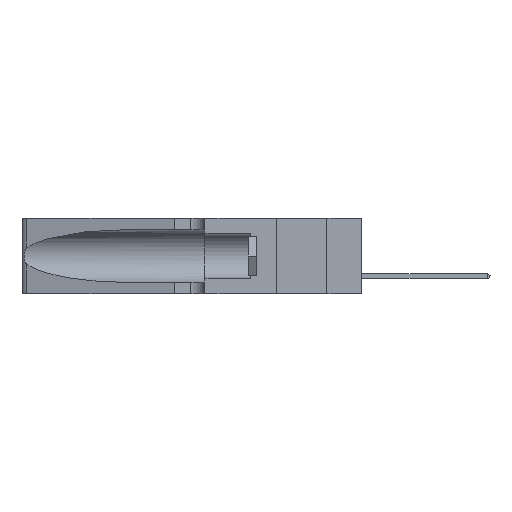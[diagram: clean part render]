
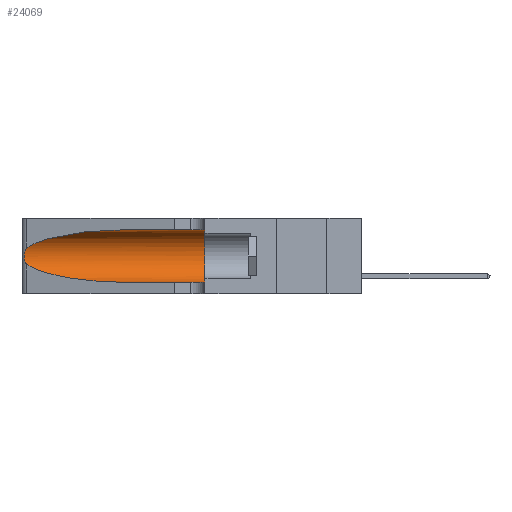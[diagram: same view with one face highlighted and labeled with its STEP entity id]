
A CAD part, left-side view. The second image highlights one B-rep face of the part: STEP entity #24069.
In plain terms, the highlighted cylindrical face has radius 3.308 mm (diameter 6.617 mm), a partial arc.
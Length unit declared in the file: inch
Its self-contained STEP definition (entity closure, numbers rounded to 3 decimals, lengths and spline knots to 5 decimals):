
#251 = CARTESIAN_POINT ( 'NONE',  ( 0.1305, 0.35, 0.05475 ) ) ;
#372 = LINE ( 'NONE', #10581, #31776 ) ;
#395 = VERTEX_POINT ( 'NONE', #18227 ) ;
#619 = CARTESIAN_POINT ( 'NONE',  ( 0.26017, 1.23833, 0.17102 ) ) ;
#1752 = VERTEX_POINT ( 'NONE', #15629 ) ;
#1945 = CARTESIAN_POINT ( 'NONE',  ( 0.25787, 1.23484, 0.2124 ) ) ;
#1964 =( BOUNDED_CURVE ( )  B_SPLINE_CURVE ( 3, ( #29571, #5136, #15035, #30301 ),
 .UNSPECIFIED., .F., .F. ) 
 B_SPLINE_CURVE_WITH_KNOTS ( ( 4, 4 ),
 ( 1.5708, 2.84003 ),
 .UNSPECIFIED. ) 
 CURVE ( )  GEOMETRIC_REPRESENTATION_ITEM ( )  RATIONAL_B_SPLINE_CURVE ( ( 1., 0.87, 0.87, 1. ) ) 
 REPRESENTATION_ITEM ( '' )  );
#4533 = ORIENTED_EDGE ( 'NONE', *, *, #20841, .F. ) ;
#4893 = VERTEX_POINT ( 'NONE', #251 ) ;
#5136 = CARTESIAN_POINT ( 'NONE',  ( 0.18966, 0.96281, 0.31525 ) ) ;
#5441 = AXIS2_PLACEMENT_3D ( 'NONE', #22650, #25826, #28469 ) ;
#7196 = CARTESIAN_POINT ( 'NONE',  ( 0.25555, 1.22994, 0.2215 ) ) ;
#7290 = DIRECTION ( 'NONE',  ( 0., -1., 0. ) ) ;
#7415 = VECTOR ( 'NONE', #7290, 39.37008 ) ;
#7799 = CARTESIAN_POINT ( 'NONE',  ( 0.25487, 1.22718, 0.14631 ) ) ;
#8104 = DIRECTION ( 'NONE',  ( 0., 1., 0. ) ) ;
#8957 = CARTESIAN_POINT ( 'NONE',  ( 0.1305, 0.72297, 0.05475 ) ) ;
#9062 = VERTEX_POINT ( 'NONE', #10924 ) ;
#9715 = VERTEX_POINT ( 'NONE', #16501 ) ;
#9868 = CYLINDRICAL_SURFACE ( 'NONE', #5441, 0.13025 ) ;
#10155 = CARTESIAN_POINT ( 'NONE',  ( 0.26018, 1.23835, 0.19895 ) ) ;
#10369 = CARTESIAN_POINT ( 'NONE',  ( 0.25639, 1.23186, 0.15144 ) ) ;
#10581 = CARTESIAN_POINT ( 'NONE',  ( 0.1305, 1.61858, 0.05475 ) ) ;
#10808 = ORIENTED_EDGE ( 'NONE', *, *, #13921, .T. ) ;
#10924 = CARTESIAN_POINT ( 'NONE',  ( 0.25487, 1.22718, 0.22369 ) ) ;
#11515 = CARTESIAN_POINT ( 'NONE',  ( 0.18966, 0.96281, 0.05475 ) ) ;
#12256 = B_SPLINE_CURVE_WITH_KNOTS ( 'NONE', 3,
 ( #16775, #7196, #29017, #1945, #22813, #10155, #22604, #27785, #619, #30407, #27897, #10369, #12957, #7799 ),
 .UNSPECIFIED., .F., .F.,
 ( 4, 2, 2, 2, 2, 2, 4 ),
 ( 0., 0.00027, 0.00053, 0.00107, 0.0016, 0.00187, 0.00214 ),
 .UNSPECIFIED. ) ;
#12534 = CARTESIAN_POINT ( 'NONE',  ( 0.1305, 1.61858, 0.31525 ) ) ;
#12957 = CARTESIAN_POINT ( 'NONE',  ( 0.25555, 1.22993, 0.14849 ) ) ;
#13382 = DIRECTION ( 'NONE',  ( 0., -1., 0. ) ) ;
#13627 = EDGE_CURVE ( 'NONE', #395, #9062, #1964, .T. ) ;
#13921 = EDGE_CURVE ( 'NONE', #1752, #9715, #23591, .T. ) ;
#14079 = CARTESIAN_POINT ( 'NONE',  ( 0.1305, 0.35, 0.31525 ) ) ;
#15035 = CARTESIAN_POINT ( 'NONE',  ( 0.2373, 1.15595, 0.28018 ) ) ;
#15629 = CARTESIAN_POINT ( 'NONE',  ( 0.25487, 1.22718, 0.14631 ) ) ;
#16501 = CARTESIAN_POINT ( 'NONE',  ( 0.1305, 0.72297, 0.05475 ) ) ;
#16662 = VERTEX_POINT ( 'NONE', #14079 ) ;
#16775 = CARTESIAN_POINT ( 'NONE',  ( 0.25487, 1.22718, 0.22369 ) ) ;
#17784 = ORIENTED_EDGE ( 'NONE', *, *, #29900, .T. ) ;
#18227 = CARTESIAN_POINT ( 'NONE',  ( 0.1305, 0.72297, 0.31525 ) ) ;
#18666 = DIRECTION ( 'NONE',  ( 0., 0., 1. ) ) ;
#20630 = EDGE_CURVE ( 'NONE', #9715, #4893, #372, .T. ) ;
#20841 = EDGE_CURVE ( 'NONE', #395, #16662, #22850, .T. ) ;
#21271 = CARTESIAN_POINT ( 'NONE',  ( 0.25487, 1.22718, 0.14631 ) ) ;
#22589 = CIRCLE ( 'NONE', #29714, 0.13025 ) ;
#22604 = CARTESIAN_POINT ( 'NONE',  ( 0.26075, 1.23896, 0.19203 ) ) ;
#22650 = CARTESIAN_POINT ( 'NONE',  ( 0.1305, 1.61858, 0.185 ) ) ;
#22813 = CARTESIAN_POINT ( 'NONE',  ( 0.25854, 1.2359, 0.20912 ) ) ;
#22850 = LINE ( 'NONE', #12534, #7415 ) ;
#22991 = FACE_OUTER_BOUND ( 'NONE', #29648, .T. ) ;
#23337 = CARTESIAN_POINT ( 'NONE',  ( 0.1305, 0.35, 0.185 ) ) ;
#23591 =( BOUNDED_CURVE ( )  B_SPLINE_CURVE ( 3, ( #21271, #23771, #11515, #8957 ),
 .UNSPECIFIED., .F., .T. ) 
 B_SPLINE_CURVE_WITH_KNOTS ( ( 4, 4 ),
 ( 3.44316, 4.71239 ),
 .UNSPECIFIED. ) 
 CURVE ( )  GEOMETRIC_REPRESENTATION_ITEM ( )  RATIONAL_B_SPLINE_CURVE ( ( 1., 0.87, 0.87, 1. ) ) 
 REPRESENTATION_ITEM ( '' )  );
#23753 = ORIENTED_EDGE ( 'NONE', *, *, #13627, .T. ) ;
#23771 = CARTESIAN_POINT ( 'NONE',  ( 0.2373, 1.15595, 0.08982 ) ) ;
#23915 = EDGE_CURVE ( 'NONE', #16662, #4893, #22589, .T. ) ;
#24069 = ADVANCED_FACE ( 'NONE', ( #22991 ), #9868, .F. ) ;
#25826 = DIRECTION ( 'NONE',  ( 0., -1., 0. ) ) ;
#26254 = ORIENTED_EDGE ( 'NONE', *, *, #20630, .T. ) ;
#27785 = CARTESIAN_POINT ( 'NONE',  ( 0.26075, 1.23896, 0.178 ) ) ;
#27897 = CARTESIAN_POINT ( 'NONE',  ( 0.25789, 1.23486, 0.15765 ) ) ;
#28469 = DIRECTION ( 'NONE',  ( 0., 0., -1. ) ) ;
#29017 = CARTESIAN_POINT ( 'NONE',  ( 0.25639, 1.23184, 0.21858 ) ) ;
#29571 = CARTESIAN_POINT ( 'NONE',  ( 0.1305, 0.72297, 0.31525 ) ) ;
#29648 = EDGE_LOOP ( 'NONE', ( #23753, #17784, #10808, #26254, #30387, #4533 ) ) ;
#29714 = AXIS2_PLACEMENT_3D ( 'NONE', #23337, #8104, #18666 ) ;
#29900 = EDGE_CURVE ( 'NONE', #9062, #1752, #12256, .T. ) ;
#30301 = CARTESIAN_POINT ( 'NONE',  ( 0.25487, 1.22718, 0.22369 ) ) ;
#30387 = ORIENTED_EDGE ( 'NONE', *, *, #23915, .F. ) ;
#30407 = CARTESIAN_POINT ( 'NONE',  ( 0.25856, 1.23593, 0.16098 ) ) ;
#31776 = VECTOR ( 'NONE', #13382, 39.37008 ) ;
